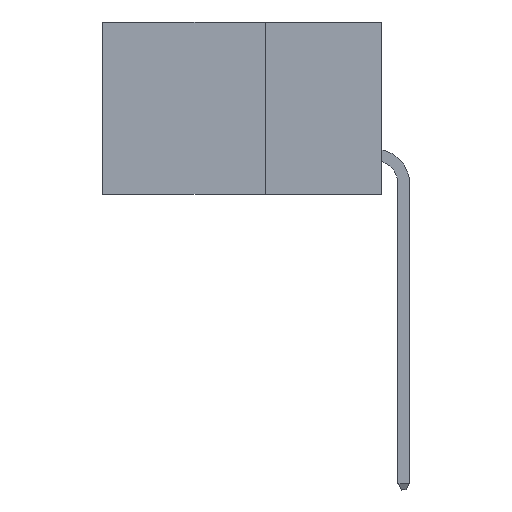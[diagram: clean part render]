
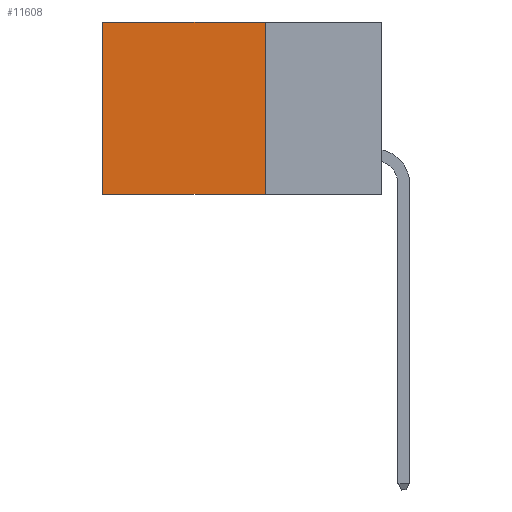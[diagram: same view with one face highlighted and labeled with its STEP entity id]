
A CAD part, left-side view. The second image highlights one B-rep face of the part: STEP entity #11608.
In plain terms, the highlighted planar face has unit normal (-1, 0, 0).
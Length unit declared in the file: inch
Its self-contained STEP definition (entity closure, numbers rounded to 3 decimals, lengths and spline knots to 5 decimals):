
#105 = EDGE_LOOP ( 'NONE', ( #5820, #4271, #21645, #17067 ) ) ;
#589 = CARTESIAN_POINT ( 'NONE',  ( 0.2875, 0.25, 0. ) ) ;
#755 = LINE ( 'NONE', #1967, #7869 ) ;
#1167 = CARTESIAN_POINT ( 'NONE',  ( 0.2875, 0.6, 0. ) ) ;
#1967 = CARTESIAN_POINT ( 'NONE',  ( 0.2875, 0.25, 0. ) ) ;
#2811 = CARTESIAN_POINT ( 'NONE',  ( 0.2875, 0.25, -0.37 ) ) ;
#3834 = VECTOR ( 'NONE', #12321, 39.37008 ) ;
#4271 = ORIENTED_EDGE ( 'NONE', *, *, #21646, .F. ) ;
#4893 = LINE ( 'NONE', #589, #3834 ) ;
#5358 = CARTESIAN_POINT ( 'NONE',  ( 0.2875, 0.6, 0. ) ) ;
#5530 = DIRECTION ( 'NONE',  ( 1., 0., 0. ) ) ;
#5820 = ORIENTED_EDGE ( 'NONE', *, *, #18682, .T. ) ;
#5830 = EDGE_CURVE ( 'NONE', #16372, #15043, #755, .T. ) ;
#6465 = CARTESIAN_POINT ( 'NONE',  ( 0.2875, 0.6, -0.37 ) ) ;
#7869 = VECTOR ( 'NONE', #15535, 39.37008 ) ;
#7923 = VECTOR ( 'NONE', #18703, 39.37008 ) ;
#7946 = VECTOR ( 'NONE', #9550, 39.37008 ) ;
#8421 = LINE ( 'NONE', #5358, #7923 ) ;
#9550 = DIRECTION ( 'NONE',  ( 0., 1., 0. ) ) ;
#9681 = PLANE ( 'NONE',  #21080 ) ;
#11608 = ADVANCED_FACE ( 'NONE', ( #21055 ), #9681, .F. ) ;
#12321 = DIRECTION ( 'NONE',  ( 0., 0., -1. ) ) ;
#13889 = CARTESIAN_POINT ( 'NONE',  ( 0.2875, 0.25, -0.37 ) ) ;
#15043 = VERTEX_POINT ( 'NONE', #1167 ) ;
#15535 = DIRECTION ( 'NONE',  ( 0., 1., 0. ) ) ;
#16371 = VERTEX_POINT ( 'NONE', #13889 ) ;
#16372 = VERTEX_POINT ( 'NONE', #17333 ) ;
#17067 = ORIENTED_EDGE ( 'NONE', *, *, #5830, .T. ) ;
#17333 = CARTESIAN_POINT ( 'NONE',  ( 0.2875, 0.25, 0. ) ) ;
#18682 = EDGE_CURVE ( 'NONE', #15043, #19557, #8421, .T. ) ;
#18703 = DIRECTION ( 'NONE',  ( 0., 0., -1. ) ) ;
#19557 = VERTEX_POINT ( 'NONE', #6465 ) ;
#19703 = DIRECTION ( 'NONE',  ( 0., 0., -1. ) ) ;
#20199 = CARTESIAN_POINT ( 'NONE',  ( 0.2875, 0.25, 0. ) ) ;
#20789 = LINE ( 'NONE', #2811, #7946 ) ;
#20991 = EDGE_CURVE ( 'NONE', #16372, #16371, #4893, .T. ) ;
#21055 = FACE_OUTER_BOUND ( 'NONE', #105, .T. ) ;
#21080 = AXIS2_PLACEMENT_3D ( 'NONE', #20199, #5530, #19703 ) ;
#21645 = ORIENTED_EDGE ( 'NONE', *, *, #20991, .F. ) ;
#21646 = EDGE_CURVE ( 'NONE', #16371, #19557, #20789, .T. ) ;
